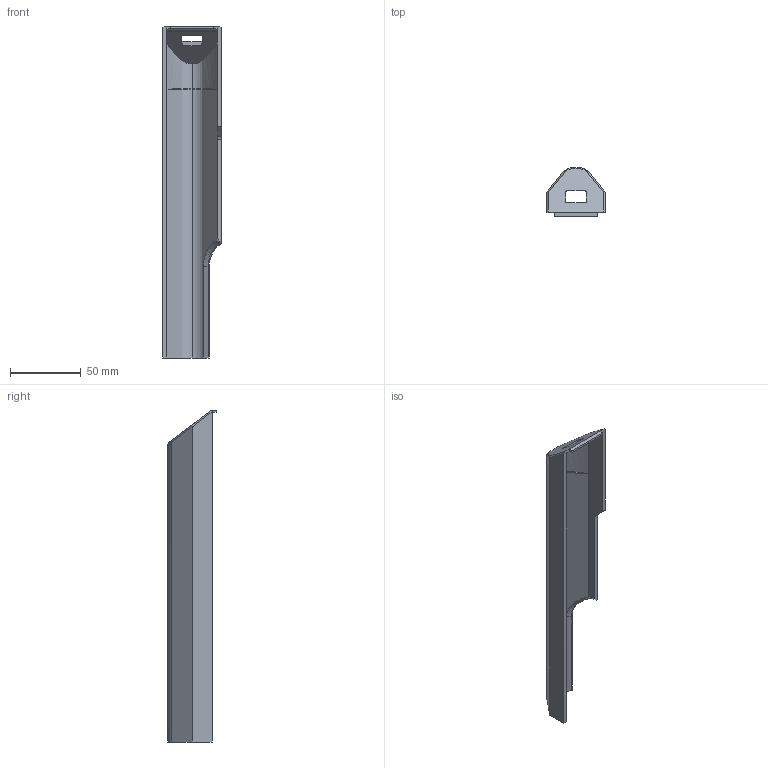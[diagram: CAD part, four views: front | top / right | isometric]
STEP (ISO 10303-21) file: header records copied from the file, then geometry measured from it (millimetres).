
FILE_DESCRIPTION(/* description */ (''),/* implementation_level */ '2;1');
FILE_NAME(/* name */ 'Printed Dust Cover - v3.0 Spec.stp',/* time_stamp */ '2022-03-21T12:35:28-05:00',/* author */ ('johne'),/* organization */ (''),/* preprocessor_version */ 'ST-DEVELOPER v18.1',/* originating_system */ 'Autodesk Inventor 2020',/* authorisation */ '');
FILE_SCHEMA (('AUTOMOTIVE_DESIGN { 1 0 10303 214 3 1 1 }'));
Length unit declared in the file: millimetre
Products named in the file (1): Printed Dust Cover - v3.0 Spec
Bounding box: 41.43 x 34.27 x 235.11 mm (x, y, z)
Volume: 37833.8 mm3; surface area: 34150.8 mm2
Topology: 1 solids, 1 shells, 56 faces, 153 edges, 99 vertices
Faces by surface type: plane 35, cylinder 15, cone 3, bspline 3
Entity records: 2077 total; most frequent: CARTESIAN_POINT 610, ORIENTED_EDGE 306, DIRECTION 284, EDGE_CURVE 153, VERTEX_POINT 99, LINE 98, VECTOR 98, AXIS2_PLACEMENT_3D 93
